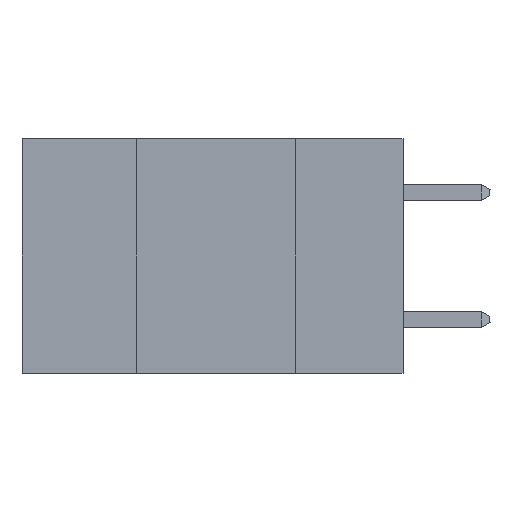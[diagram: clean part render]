
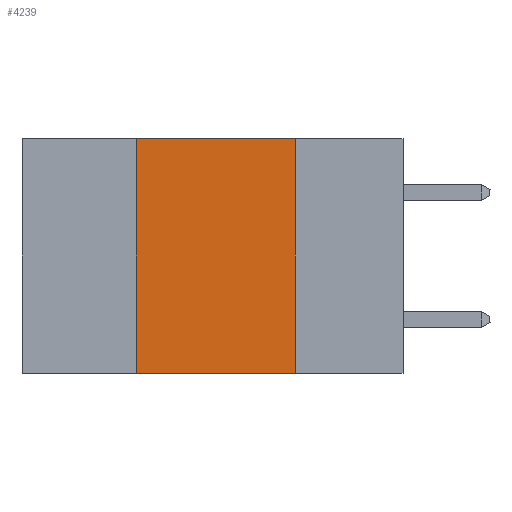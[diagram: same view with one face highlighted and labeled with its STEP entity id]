
A CAD part, left-side view. The second image highlights one B-rep face of the part: STEP entity #4239.
In plain terms, the highlighted planar face has unit normal (-1, 0, 0).
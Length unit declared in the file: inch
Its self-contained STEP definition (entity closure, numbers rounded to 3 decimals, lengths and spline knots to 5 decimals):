
#810 = VECTOR ( 'NONE', #2374, 39.37008 ) ;
#1568 = EDGE_CURVE ( 'NONE', #17214, #10189, #4310, .T. ) ;
#1667 = DIRECTION ( 'NONE',  ( 0., -1., 0. ) ) ;
#1966 = FACE_OUTER_BOUND ( 'NONE', #10206, .T. ) ;
#2374 = DIRECTION ( 'NONE',  ( 0., 0., -1. ) ) ;
#2538 = VECTOR ( 'NONE', #1667, 39.37008 ) ;
#3345 = VECTOR ( 'NONE', #19491, 39.37008 ) ;
#3898 = VERTEX_POINT ( 'NONE', #11542 ) ;
#4239 = ADVANCED_FACE ( 'NONE', ( #1966 ), #12294, .F. ) ;
#4310 = LINE ( 'NONE', #34237, #3345 ) ;
#4919 = CARTESIAN_POINT ( 'NONE',  ( 0., 0.42, 0. ) ) ;
#5417 = CARTESIAN_POINT ( 'NONE',  ( 0., 0.42, 0. ) ) ;
#10189 = VERTEX_POINT ( 'NONE', #21173 ) ;
#10206 = EDGE_LOOP ( 'NONE', ( #37411, #13744, #37625, #29003 ) ) ;
#11205 = DIRECTION ( 'NONE',  ( 0., 0., 1. ) ) ;
#11542 = CARTESIAN_POINT ( 'NONE',  ( 0., 0.17, 0. ) ) ;
#12294 = PLANE ( 'NONE',  #20845 ) ;
#13744 = ORIENTED_EDGE ( 'NONE', *, *, #28744, .F. ) ;
#14953 = CARTESIAN_POINT ( 'NONE',  ( 0., 0.6, 0. ) ) ;
#16541 = LINE ( 'NONE', #4919, #33503 ) ;
#17214 = VERTEX_POINT ( 'NONE', #21536 ) ;
#17888 = CARTESIAN_POINT ( 'NONE',  ( 0., 0.17, 0. ) ) ;
#19491 = DIRECTION ( 'NONE',  ( 0., -1., 0. ) ) ;
#20845 = AXIS2_PLACEMENT_3D ( 'NONE', #14953, #27299, #35997 ) ;
#21173 = CARTESIAN_POINT ( 'NONE',  ( 0., 0.17, -0.37 ) ) ;
#21536 = CARTESIAN_POINT ( 'NONE',  ( 0., 0.42, -0.37 ) ) ;
#23901 = LINE ( 'NONE', #17888, #810 ) ;
#27055 = EDGE_CURVE ( 'NONE', #3898, #10189, #23901, .T. ) ;
#27299 = DIRECTION ( 'NONE',  ( 1., 0., 0. ) ) ;
#28744 = EDGE_CURVE ( 'NONE', #35587, #3898, #29831, .T. ) ;
#29003 = ORIENTED_EDGE ( 'NONE', *, *, #1568, .T. ) ;
#29831 = LINE ( 'NONE', #37532, #2538 ) ;
#33503 = VECTOR ( 'NONE', #11205, 39.37008 ) ;
#34237 = CARTESIAN_POINT ( 'NONE',  ( 0., 0.6, -0.37 ) ) ;
#35587 = VERTEX_POINT ( 'NONE', #5417 ) ;
#35997 = DIRECTION ( 'NONE',  ( 0., 0., -1. ) ) ;
#37312 = EDGE_CURVE ( 'NONE', #17214, #35587, #16541, .T. ) ;
#37411 = ORIENTED_EDGE ( 'NONE', *, *, #27055, .F. ) ;
#37532 = CARTESIAN_POINT ( 'NONE',  ( 0., 0.6, 0. ) ) ;
#37625 = ORIENTED_EDGE ( 'NONE', *, *, #37312, .F. ) ;
